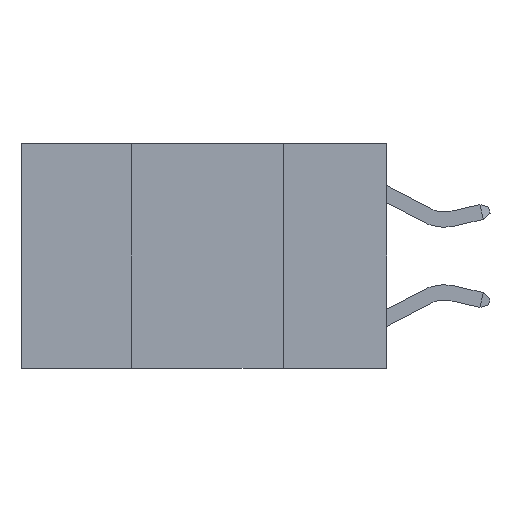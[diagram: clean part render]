
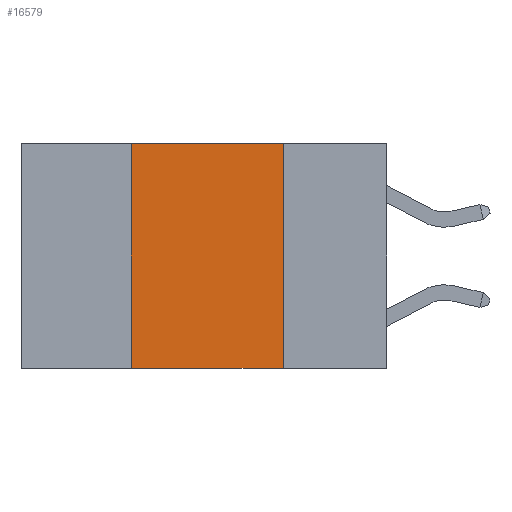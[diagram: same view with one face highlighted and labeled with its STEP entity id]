
A CAD part, left-side view. The second image highlights one B-rep face of the part: STEP entity #16579.
In plain terms, the highlighted planar face has unit normal (-1, 0, 0).
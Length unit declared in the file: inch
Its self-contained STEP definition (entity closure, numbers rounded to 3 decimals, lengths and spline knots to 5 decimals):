
#1692 = VECTOR ( 'NONE', #7575, 39.37008 ) ;
#1693 = LINE ( 'NONE', #14127, #5369 ) ;
#2402 = VERTEX_POINT ( 'NONE', #4996 ) ;
#3008 = ORIENTED_EDGE ( 'NONE', *, *, #7466, .F. ) ;
#3681 = VECTOR ( 'NONE', #18089, 39.37008 ) ;
#4414 = CARTESIAN_POINT ( 'NONE',  ( 0., 0.6, 0. ) ) ;
#4996 = CARTESIAN_POINT ( 'NONE',  ( 0., 0.42, -0.37 ) ) ;
#5030 = DIRECTION ( 'NONE',  ( 0., 0., -1. ) ) ;
#5050 = CARTESIAN_POINT ( 'NONE',  ( 0., 0.6, -0.37 ) ) ;
#5052 = EDGE_CURVE ( 'NONE', #18742, #5288, #1693, .T. ) ;
#5157 = ORIENTED_EDGE ( 'NONE', *, *, #15139, .F. ) ;
#5288 = VERTEX_POINT ( 'NONE', #14635 ) ;
#5369 = VECTOR ( 'NONE', #5030, 39.37008 ) ;
#6094 = CARTESIAN_POINT ( 'NONE',  ( 0., 0.6, 0. ) ) ;
#7466 = EDGE_CURVE ( 'NONE', #15519, #18742, #15868, .T. ) ;
#7575 = DIRECTION ( 'NONE',  ( 0., 0., 1. ) ) ;
#9232 = PLANE ( 'NONE',  #20017 ) ;
#9626 = DIRECTION ( 'NONE',  ( 0., -1., 0. ) ) ;
#9937 = LINE ( 'NONE', #12037, #1692 ) ;
#9954 = ORIENTED_EDGE ( 'NONE', *, *, #11309, .T. ) ;
#10754 = DIRECTION ( 'NONE',  ( 0., 0., -1. ) ) ;
#11309 = EDGE_CURVE ( 'NONE', #2402, #5288, #18859, .T. ) ;
#12037 = CARTESIAN_POINT ( 'NONE',  ( 0., 0.42, 0. ) ) ;
#14127 = CARTESIAN_POINT ( 'NONE',  ( 0., 0.17, 0. ) ) ;
#14635 = CARTESIAN_POINT ( 'NONE',  ( 0., 0.17, -0.37 ) ) ;
#15139 = EDGE_CURVE ( 'NONE', #2402, #15519, #9937, .T. ) ;
#15519 = VERTEX_POINT ( 'NONE', #19015 ) ;
#15744 = VECTOR ( 'NONE', #9626, 39.37008 ) ;
#15868 = LINE ( 'NONE', #4414, #3681 ) ;
#16360 = ORIENTED_EDGE ( 'NONE', *, *, #5052, .F. ) ;
#16499 = FACE_OUTER_BOUND ( 'NONE', #16662, .T. ) ;
#16579 = ADVANCED_FACE ( 'NONE', ( #16499 ), #9232, .F. ) ;
#16662 = EDGE_LOOP ( 'NONE', ( #16360, #3008, #5157, #9954 ) ) ;
#18089 = DIRECTION ( 'NONE',  ( 0., -1., 0. ) ) ;
#18742 = VERTEX_POINT ( 'NONE', #18921 ) ;
#18859 = LINE ( 'NONE', #5050, #15744 ) ;
#18921 = CARTESIAN_POINT ( 'NONE',  ( 0., 0.17, 0. ) ) ;
#19015 = CARTESIAN_POINT ( 'NONE',  ( 0., 0.42, 0. ) ) ;
#19901 = DIRECTION ( 'NONE',  ( 1., 0., 0. ) ) ;
#20017 = AXIS2_PLACEMENT_3D ( 'NONE', #6094, #19901, #10754 ) ;
